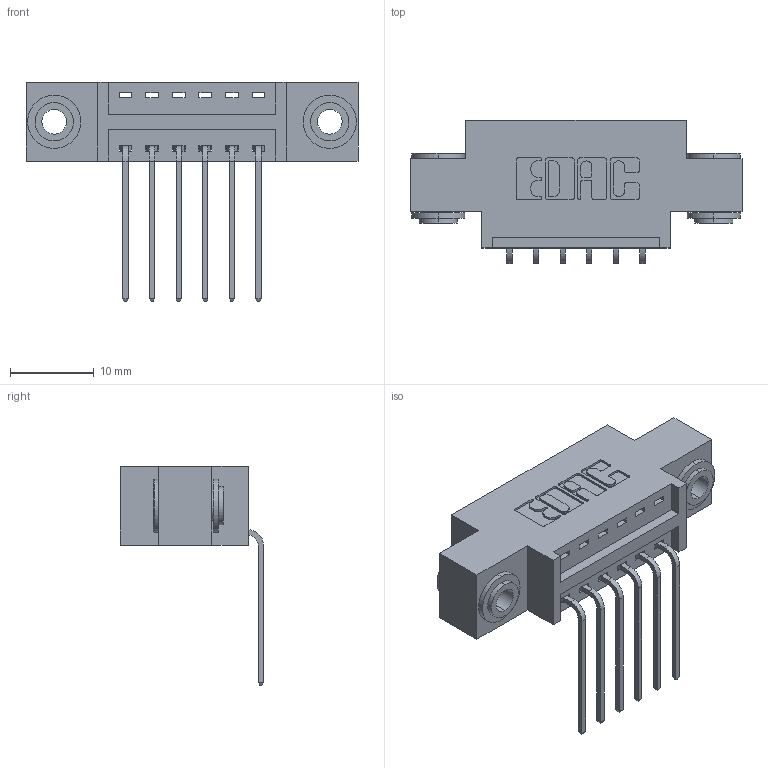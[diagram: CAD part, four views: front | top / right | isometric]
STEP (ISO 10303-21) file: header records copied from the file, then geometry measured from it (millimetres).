
FILE_DESCRIPTION (( 'STEP AP203' ), '1' );
FILE_NAME ('346-006-559-603.STEP', '2022-05-04T19:16:39', ( '' ), ( '' ), 'SwSTEP 2.0', 'SolidWorks 2020', '' );
FILE_SCHEMA (( 'CONFIG_CONTROL_DESIGN' ));
Length unit declared in the file: inch
Products named in the file (4): 345-250-002_345-250-002-102; 346 Part_0.170 Offset - 0.156 Dia-TH; 346-006-559-603; 345-292-001_558 559 Tail - 1
Assembly tree (9 placements, depth 2):
  346-006-559-603
    346 Part_0.170 Offset - 0.156 Dia-TH
    345-292-001_558 559 Tail - 1  x6
    345-250-002_345-250-002-102  x2
Bounding box: 39.62 x 17.08 x 26.16 mm (x, y, z)
Volume: 3411.5 mm3; surface area: 4406.6 mm2
Topology: 9 solids, 9 shells, 538 faces, 1545 edges, 1018 vertices
Faces by surface type: plane 356, cylinder 174, cone 8
Entity records: 9852 total; most frequent: CARTESIAN_POINT 1683, ORIENTED_EDGE 1614, DIRECTION 1557, EDGE_CURVE 807, VECTOR 627, LINE 627, VERTEX_POINT 534, AXIS2_PLACEMENT_3D 465
